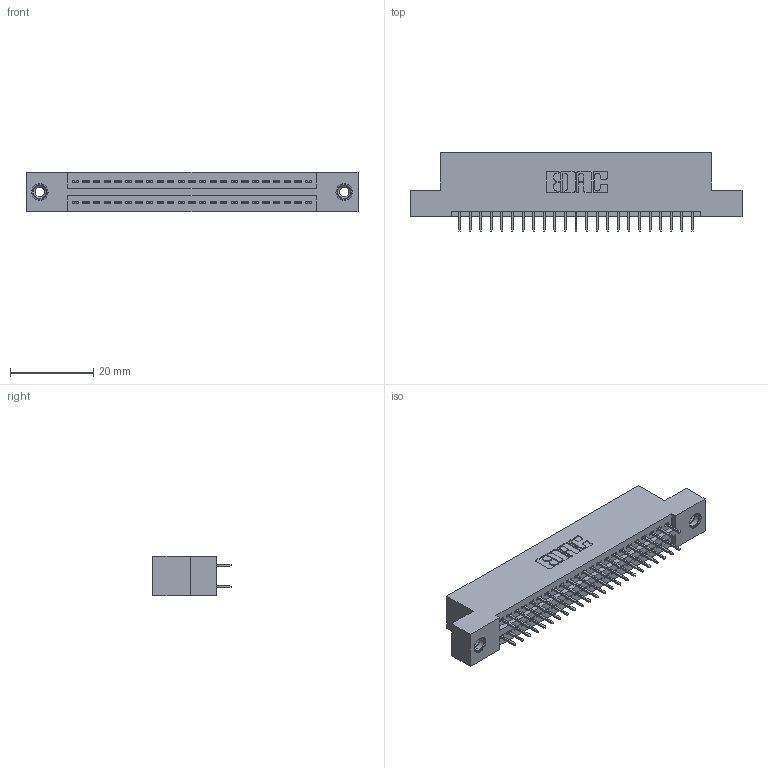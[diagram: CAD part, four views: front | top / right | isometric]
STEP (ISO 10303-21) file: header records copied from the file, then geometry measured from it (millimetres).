
FILE_DESCRIPTION (( 'STEP AP203' ), '1' );
FILE_NAME ('895-046-525-208.STEP', '2020-09-27T05:22:27', ( '' ), ( '' ), 'SwSTEP 2.0', 'SolidWorks 2020', '' );
FILE_SCHEMA (( 'CONFIG_CONTROL_DESIGN' ));
Length unit declared in the file: inch
Products named in the file (4): 345-250-001_345-250-003-102; 845 Part_Flush Mounting Lugs - 0.156 Dia-TI; 345-292-001_345-293-125; 895-046-525-208
Assembly tree (49 placements, depth 2):
  895-046-525-208
    845 Part_Flush Mounting Lugs - 0.156 Dia-TI
    345-292-001_345-293-125  x46
    345-250-001_345-250-003-102  x2
Bounding box: 79.63 x 18.72 x 9.4 mm (x, y, z)
Volume: 7476.6 mm3; surface area: 10469 mm2
Topology: 49 solids, 49 shells, 2670 faces, 7515 edges, 4818 vertices
Faces by surface type: plane 1906, cylinder 748, cone 12, torus 4
Entity records: 21864 total; most frequent: CARTESIAN_POINT 3663, ORIENTED_EDGE 3590, DIRECTION 3281, EDGE_CURVE 1795, LINE 1555, VECTOR 1555, VERTEX_POINT 1188, AXIS2_PLACEMENT_3D 863
